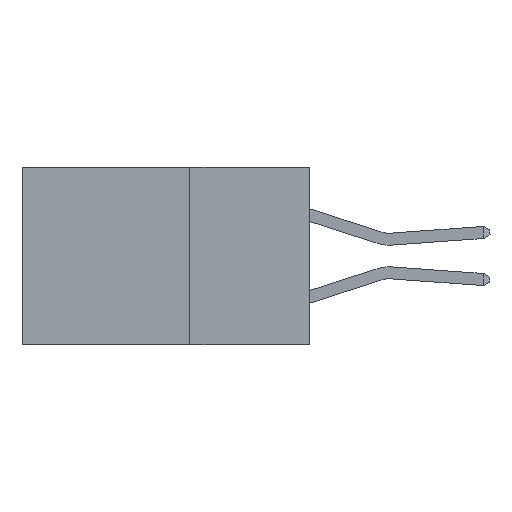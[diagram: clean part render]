
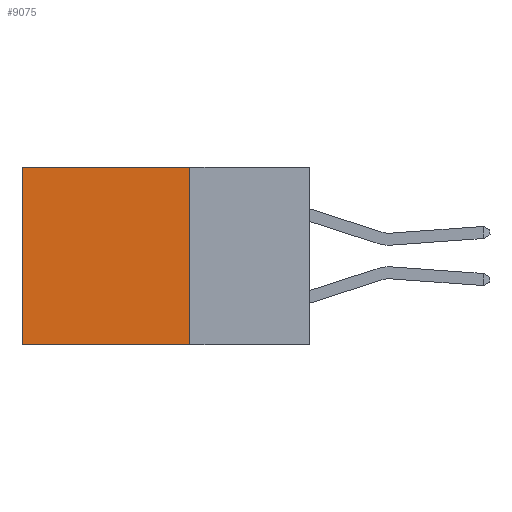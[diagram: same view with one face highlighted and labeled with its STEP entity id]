
A CAD part, left-side view. The second image highlights one B-rep face of the part: STEP entity #9075.
In plain terms, the highlighted planar face has unit normal (-1, 0, 0).
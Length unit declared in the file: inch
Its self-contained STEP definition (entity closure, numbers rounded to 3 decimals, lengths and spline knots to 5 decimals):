
#822 = EDGE_CURVE ( 'NONE', #7218, #5292, #8919, .T. ) ;
#832 = ORIENTED_EDGE ( 'NONE', *, *, #8620, .T. ) ;
#1983 = CARTESIAN_POINT ( 'NONE',  ( 0.298, 0.6, 0. ) ) ;
#2287 = CARTESIAN_POINT ( 'NONE',  ( 0.298, 0.6, -0.37 ) ) ;
#2650 = EDGE_LOOP ( 'NONE', ( #6106, #3454, #12045, #832 ) ) ;
#3094 = DIRECTION ( 'NONE',  ( 0., 0., -1. ) ) ;
#3116 = VECTOR ( 'NONE', #10826, 39.37008 ) ;
#3454 = ORIENTED_EDGE ( 'NONE', *, *, #4409, .F. ) ;
#4409 = EDGE_CURVE ( 'NONE', #5292, #9827, #12814, .T. ) ;
#5075 = DIRECTION ( 'NONE',  ( 0., 1., 0. ) ) ;
#5292 = VERTEX_POINT ( 'NONE', #10596 ) ;
#5324 = CARTESIAN_POINT ( 'NONE',  ( 0.298, 0.25, 0. ) ) ;
#5947 = DIRECTION ( 'NONE',  ( 0., 1., 0. ) ) ;
#5994 = CARTESIAN_POINT ( 'NONE',  ( 0.298, 0.25, 0. ) ) ;
#6106 = ORIENTED_EDGE ( 'NONE', *, *, #12036, .T. ) ;
#6644 = CARTESIAN_POINT ( 'NONE',  ( 0.298, 0.25, -0.37 ) ) ;
#6727 = LINE ( 'NONE', #5994, #11988 ) ;
#6944 = VECTOR ( 'NONE', #5075, 39.37008 ) ;
#7218 = VERTEX_POINT ( 'NONE', #5324 ) ;
#7244 = FACE_OUTER_BOUND ( 'NONE', #2650, .T. ) ;
#7470 = VECTOR ( 'NONE', #3094, 39.37008 ) ;
#7495 = VERTEX_POINT ( 'NONE', #11557 ) ;
#8620 = EDGE_CURVE ( 'NONE', #7218, #7495, #6727, .T. ) ;
#8919 = LINE ( 'NONE', #9871, #3116 ) ;
#9075 = ADVANCED_FACE ( 'NONE', ( #7244 ), #11011, .F. ) ;
#9827 = VERTEX_POINT ( 'NONE', #2287 ) ;
#9871 = CARTESIAN_POINT ( 'NONE',  ( 0.298, 0.25, 0. ) ) ;
#10021 = AXIS2_PLACEMENT_3D ( 'NONE', #10888, #10822, #10602 ) ;
#10596 = CARTESIAN_POINT ( 'NONE',  ( 0.298, 0.25, -0.37 ) ) ;
#10602 = DIRECTION ( 'NONE',  ( 0., 0., -1. ) ) ;
#10822 = DIRECTION ( 'NONE',  ( 1., 0., 0. ) ) ;
#10826 = DIRECTION ( 'NONE',  ( 0., 0., -1. ) ) ;
#10888 = CARTESIAN_POINT ( 'NONE',  ( 0.298, 0.25, 0. ) ) ;
#11011 = PLANE ( 'NONE',  #10021 ) ;
#11557 = CARTESIAN_POINT ( 'NONE',  ( 0.298, 0.6, 0. ) ) ;
#11988 = VECTOR ( 'NONE', #5947, 39.37008 ) ;
#12036 = EDGE_CURVE ( 'NONE', #7495, #9827, #13316, .T. ) ;
#12045 = ORIENTED_EDGE ( 'NONE', *, *, #822, .F. ) ;
#12814 = LINE ( 'NONE', #6644, #6944 ) ;
#13316 = LINE ( 'NONE', #1983, #7470 ) ;
